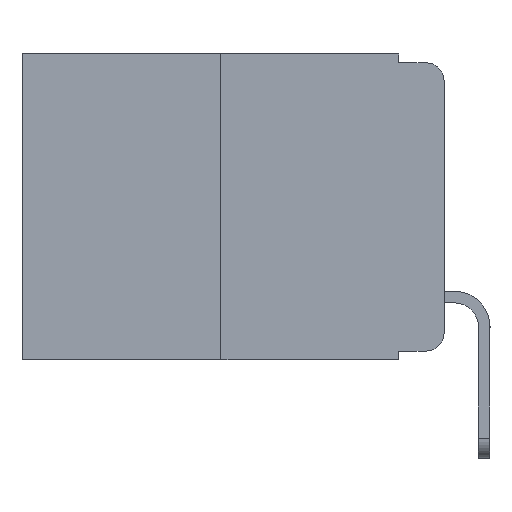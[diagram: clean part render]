
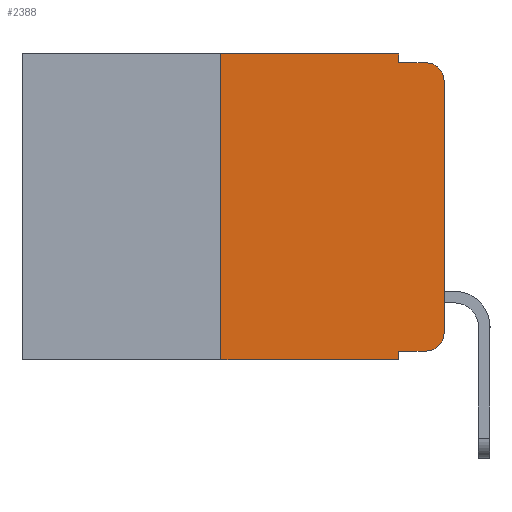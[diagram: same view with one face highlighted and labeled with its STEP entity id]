
A CAD part, left-side view. The second image highlights one B-rep face of the part: STEP entity #2388.
In plain terms, the highlighted planar face has unit normal (-1, 0, 0).
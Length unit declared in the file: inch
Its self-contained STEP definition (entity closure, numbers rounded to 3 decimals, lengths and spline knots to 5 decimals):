
#99 = ORIENTED_EDGE ( 'NONE', *, *, #1184, .F. ) ;
#116 = EDGE_CURVE ( 'NONE', #11575, #3623, #1819, .T. ) ;
#667 = CARTESIAN_POINT ( 'NONE',  ( 0., 0.051, 0. ) ) ;
#725 = VERTEX_POINT ( 'NONE', #13322 ) ;
#796 = CARTESIAN_POINT ( 'NONE',  ( 0., 0.051, -0.333 ) ) ;
#1184 = EDGE_CURVE ( 'NONE', #3623, #5239, #16648, .T. ) ;
#1247 = ORIENTED_EDGE ( 'NONE', *, *, #13387, .F. ) ;
#1819 = LINE ( 'NONE', #10916, #13455 ) ;
#1962 = ORIENTED_EDGE ( 'NONE', *, *, #2219, .T. ) ;
#2219 = EDGE_CURVE ( 'NONE', #9069, #5239, #11444, .T. ) ;
#2359 = ORIENTED_EDGE ( 'NONE', *, *, #10803, .T. ) ;
#2388 = ADVANCED_FACE ( 'NONE', ( #9026 ), #10688, .F. ) ;
#2501 = VECTOR ( 'NONE', #8340, 39.37008 ) ;
#3110 = DIRECTION ( 'NONE',  ( 0., -1., 0. ) ) ;
#3257 = EDGE_CURVE ( 'NONE', #9638, #9069, #5469, .T. ) ;
#3303 = DIRECTION ( 'NONE',  ( 0., 0., 1. ) ) ;
#3623 = VERTEX_POINT ( 'NONE', #8156 ) ;
#3803 = ORIENTED_EDGE ( 'NONE', *, *, #10609, .F. ) ;
#3982 = LINE ( 'NONE', #8370, #17411 ) ;
#4043 = CARTESIAN_POINT ( 'NONE',  ( 0., 0.051, -0.333 ) ) ;
#4501 = EDGE_CURVE ( 'NONE', #8445, #11085, #8539, .T. ) ;
#4697 = ORIENTED_EDGE ( 'NONE', *, *, #4501, .T. ) ;
#4996 = VECTOR ( 'NONE', #15113, 39.37008 ) ;
#5239 = VERTEX_POINT ( 'NONE', #6734 ) ;
#5469 = LINE ( 'NONE', #15966, #2501 ) ;
#5825 = CARTESIAN_POINT ( 'NONE',  ( 0., 0.25, -0.343 ) ) ;
#6103 = CARTESIAN_POINT ( 'NONE',  ( 0., 0.473, -0.343 ) ) ;
#6116 = CARTESIAN_POINT ( 'NONE',  ( 0., 0.25, 0. ) ) ;
#6426 = CARTESIAN_POINT ( 'NONE',  ( 0., 0.02, -0.333 ) ) ;
#6734 = CARTESIAN_POINT ( 'NONE',  ( 0., 0.02, -0.01 ) ) ;
#6754 = ORIENTED_EDGE ( 'NONE', *, *, #116, .F. ) ;
#6883 = ORIENTED_EDGE ( 'NONE', *, *, #11672, .T. ) ;
#7402 = VERTEX_POINT ( 'NONE', #6426 ) ;
#7495 = VECTOR ( 'NONE', #3110, 39.37008 ) ;
#7634 = DIRECTION ( 'NONE',  ( -1., 0., 0. ) ) ;
#8068 = VECTOR ( 'NONE', #13159, 39.37008 ) ;
#8156 = CARTESIAN_POINT ( 'NONE',  ( 0., 0.051, -0.01 ) ) ;
#8175 = DIRECTION ( 'NONE',  ( 0., 0., -1. ) ) ;
#8340 = DIRECTION ( 'NONE',  ( 0., 0., 1. ) ) ;
#8370 = CARTESIAN_POINT ( 'NONE',  ( 0., 0.051, 0. ) ) ;
#8419 = DIRECTION ( 'NONE',  ( 0., 0., -1. ) ) ;
#8445 = VERTEX_POINT ( 'NONE', #5825 ) ;
#8539 = LINE ( 'NONE', #6103, #4996 ) ;
#8575 = CARTESIAN_POINT ( 'NONE',  ( 0., 0.473, 0. ) ) ;
#8837 = DIRECTION ( 'NONE',  ( 0., 0., -1. ) ) ;
#9026 = FACE_OUTER_BOUND ( 'NONE', #9573, .T. ) ;
#9069 = VERTEX_POINT ( 'NONE', #12172 ) ;
#9282 = CARTESIAN_POINT ( 'NONE',  ( 0., 0.473, 0. ) ) ;
#9331 = ORIENTED_EDGE ( 'NONE', *, *, #3257, .T. ) ;
#9342 = CARTESIAN_POINT ( 'NONE',  ( 0., 0.051, -0.343 ) ) ;
#9503 = VERTEX_POINT ( 'NONE', #4043 ) ;
#9573 = EDGE_LOOP ( 'NONE', ( #9331, #1962, #99, #6754, #3803, #1247, #4697, #13299, #6883, #2359 ) ) ;
#9638 = VERTEX_POINT ( 'NONE', #12236 ) ;
#10595 = CARTESIAN_POINT ( 'NONE',  ( 0., 0.051, -0.01 ) ) ;
#10609 = EDGE_CURVE ( 'NONE', #725, #11575, #10874, .T. ) ;
#10688 = PLANE ( 'NONE',  #15499 ) ;
#10803 = EDGE_CURVE ( 'NONE', #7402, #9638, #15259, .T. ) ;
#10810 = DIRECTION ( 'NONE',  ( 1., 0., 0. ) ) ;
#10874 = LINE ( 'NONE', #8575, #7495 ) ;
#10916 = CARTESIAN_POINT ( 'NONE',  ( 0., 0.051, 0. ) ) ;
#11085 = VERTEX_POINT ( 'NONE', #9342 ) ;
#11444 = CIRCLE ( 'NONE', #12402, 0.02 ) ;
#11450 = LINE ( 'NONE', #796, #8068 ) ;
#11575 = VERTEX_POINT ( 'NONE', #667 ) ;
#11672 = EDGE_CURVE ( 'NONE', #9503, #7402, #11450, .T. ) ;
#12172 = CARTESIAN_POINT ( 'NONE',  ( 0., 0., -0.03 ) ) ;
#12236 = CARTESIAN_POINT ( 'NONE',  ( 0., 0., -0.313 ) ) ;
#12267 = DIRECTION ( 'NONE',  ( 0., -1., 0. ) ) ;
#12402 = AXIS2_PLACEMENT_3D ( 'NONE', #13534, #13547, #8175 ) ;
#12541 = EDGE_CURVE ( 'NONE', #9503, #11085, #3982, .T. ) ;
#13159 = DIRECTION ( 'NONE',  ( 0., -1., 0. ) ) ;
#13299 = ORIENTED_EDGE ( 'NONE', *, *, #12541, .F. ) ;
#13322 = CARTESIAN_POINT ( 'NONE',  ( 0., 0.25, 0. ) ) ;
#13387 = EDGE_CURVE ( 'NONE', #8445, #725, #16800, .T. ) ;
#13439 = VECTOR ( 'NONE', #3303, 39.37008 ) ;
#13455 = VECTOR ( 'NONE', #14160, 39.37008 ) ;
#13534 = CARTESIAN_POINT ( 'NONE',  ( 0., 0.02, -0.03 ) ) ;
#13547 = DIRECTION ( 'NONE',  ( -1., 0., 0. ) ) ;
#14160 = DIRECTION ( 'NONE',  ( 0., 0., -1. ) ) ;
#15113 = DIRECTION ( 'NONE',  ( 0., -1., 0. ) ) ;
#15141 = AXIS2_PLACEMENT_3D ( 'NONE', #15273, #7634, #16534 ) ;
#15259 = CIRCLE ( 'NONE', #15141, 0.02 ) ;
#15273 = CARTESIAN_POINT ( 'NONE',  ( 0., 0.02, -0.313 ) ) ;
#15499 = AXIS2_PLACEMENT_3D ( 'NONE', #9282, #10810, #8837 ) ;
#15966 = CARTESIAN_POINT ( 'NONE',  ( 0., 0., 0. ) ) ;
#16264 = VECTOR ( 'NONE', #12267, 39.37008 ) ;
#16534 = DIRECTION ( 'NONE',  ( 0., 0., -1. ) ) ;
#16648 = LINE ( 'NONE', #10595, #16264 ) ;
#16800 = LINE ( 'NONE', #6116, #13439 ) ;
#17411 = VECTOR ( 'NONE', #8419, 39.37008 ) ;
